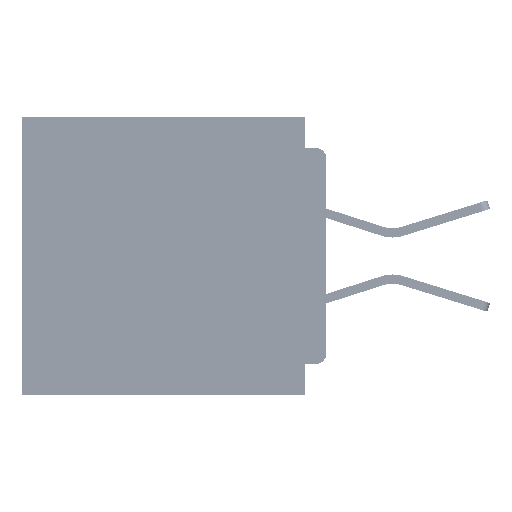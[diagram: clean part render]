
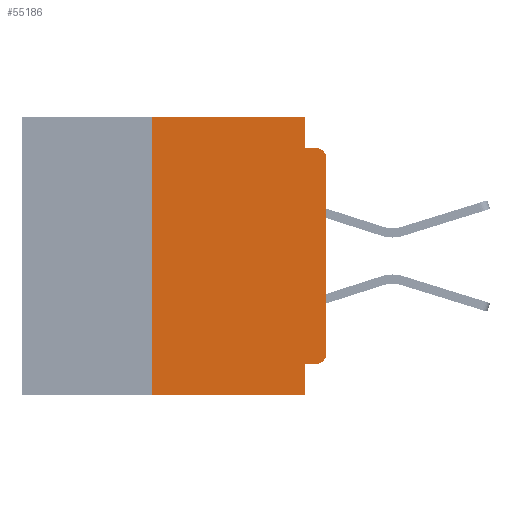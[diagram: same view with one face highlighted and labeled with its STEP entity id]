
A CAD part, left-side view. The second image highlights one B-rep face of the part: STEP entity #55186.
In plain terms, the highlighted planar face has unit normal (-1, 0, 0).
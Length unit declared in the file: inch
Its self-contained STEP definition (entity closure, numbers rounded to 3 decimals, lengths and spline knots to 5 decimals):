
#469 = EDGE_CURVE ( 'NONE', #53660, #41227, #53761, .T. ) ;
#1342 = VECTOR ( 'NONE', #25049, 39.37008 ) ;
#2038 = CARTESIAN_POINT ( 'NONE',  ( 0., 0.437, -0.4 ) ) ;
#2391 = CIRCLE ( 'NONE', #58798, 0.015 ) ;
#3403 = CIRCLE ( 'NONE', #19896, 0.015 ) ;
#4155 = DIRECTION ( 'NONE',  ( 0., -1., 0. ) ) ;
#5363 = ORIENTED_EDGE ( 'NONE', *, *, #34913, .F. ) ;
#6314 = DIRECTION ( 'NONE',  ( 1., 0., 0. ) ) ;
#6345 = ORIENTED_EDGE ( 'NONE', *, *, #62724, .F. ) ;
#6368 = VERTEX_POINT ( 'NONE', #53096 ) ;
#8986 = VERTEX_POINT ( 'NONE', #53645 ) ;
#13314 = CARTESIAN_POINT ( 'NONE',  ( 0., 0.015, -0.045 ) ) ;
#13332 = ORIENTED_EDGE ( 'NONE', *, *, #47112, .T. ) ;
#13909 = CARTESIAN_POINT ( 'NONE',  ( 0., 0.437, 0. ) ) ;
#14519 = DIRECTION ( 'NONE',  ( -1., 0., 0. ) ) ;
#14532 = LINE ( 'NONE', #15084, #1342 ) ;
#15084 = CARTESIAN_POINT ( 'NONE',  ( 0., 0., -0.355 ) ) ;
#15087 = VECTOR ( 'NONE', #4155, 39.37008 ) ;
#15425 = DIRECTION ( 'NONE',  ( -1., 0., 0. ) ) ;
#15692 = LINE ( 'NONE', #61368, #55164 ) ;
#17556 = DIRECTION ( 'NONE',  ( 0., 0., -1. ) ) ;
#18637 = ORIENTED_EDGE ( 'NONE', *, *, #59738, .F. ) ;
#18730 = EDGE_CURVE ( 'NONE', #46755, #45138, #43932, .T. ) ;
#19000 = LINE ( 'NONE', #20740, #43807 ) ;
#19896 = AXIS2_PLACEMENT_3D ( 'NONE', #44179, #14519, #49122 ) ;
#20205 = AXIS2_PLACEMENT_3D ( 'NONE', #35930, #6314, #40915 ) ;
#20740 = CARTESIAN_POINT ( 'NONE',  ( 0., 0.031, -0.4 ) ) ;
#21092 = ORIENTED_EDGE ( 'NONE', *, *, #18730, .T. ) ;
#21285 = EDGE_CURVE ( 'NONE', #45138, #56382, #3403, .T. ) ;
#21872 = DIRECTION ( 'NONE',  ( 0., -1., 0. ) ) ;
#21956 = CARTESIAN_POINT ( 'NONE',  ( 0., 0.031, -0.4 ) ) ;
#22023 = VECTOR ( 'NONE', #17556, 39.37008 ) ;
#22324 = EDGE_CURVE ( 'NONE', #53660, #56052, #59729, .T. ) ;
#23099 = DIRECTION ( 'NONE',  ( 0., 0., 1. ) ) ;
#25049 = DIRECTION ( 'NONE',  ( 0., 1., 0. ) ) ;
#25696 = CARTESIAN_POINT ( 'NONE',  ( 0., 0.25, 0. ) ) ;
#25721 = DIRECTION ( 'NONE',  ( 0., 0., -1. ) ) ;
#26771 = DIRECTION ( 'NONE',  ( 0., -1., 0. ) ) ;
#27469 = VECTOR ( 'NONE', #26771, 39.37008 ) ;
#28266 = LINE ( 'NONE', #13909, #15087 ) ;
#29336 = CARTESIAN_POINT ( 'NONE',  ( 0., 0.031, -0.045 ) ) ;
#30130 = CARTESIAN_POINT ( 'NONE',  ( 0., 0., 0. ) ) ;
#30269 = ORIENTED_EDGE ( 'NONE', *, *, #53497, .F. ) ;
#31721 = FACE_OUTER_BOUND ( 'NONE', #54273, .T. ) ;
#33463 = VECTOR ( 'NONE', #23099, 39.37008 ) ;
#34913 = EDGE_CURVE ( 'NONE', #56052, #39767, #28266, .T. ) ;
#35061 = DIRECTION ( 'NONE',  ( 0., 0., 1. ) ) ;
#35141 = LINE ( 'NONE', #42232, #22023 ) ;
#35930 = CARTESIAN_POINT ( 'NONE',  ( 0., 0.437, 0. ) ) ;
#36572 = ORIENTED_EDGE ( 'NONE', *, *, #48236, .F. ) ;
#39767 = VERTEX_POINT ( 'NONE', #54332 ) ;
#40791 = VECTOR ( 'NONE', #35061, 39.37008 ) ;
#40915 = DIRECTION ( 'NONE',  ( 0., 0., -1. ) ) ;
#41227 = VERTEX_POINT ( 'NONE', #21956 ) ;
#42232 = CARTESIAN_POINT ( 'NONE',  ( 0., 0.031, 0. ) ) ;
#43361 = CARTESIAN_POINT ( 'NONE',  ( 0., 0., -0.06 ) ) ;
#43807 = VECTOR ( 'NONE', #25721, 39.37008 ) ;
#43932 = LINE ( 'NONE', #30130, #40791 ) ;
#44179 = CARTESIAN_POINT ( 'NONE',  ( 0., 0.015, -0.06 ) ) ;
#45079 = CARTESIAN_POINT ( 'NONE',  ( 0., 0.015, -0.34 ) ) ;
#45138 = VERTEX_POINT ( 'NONE', #43361 ) ;
#45857 = ORIENTED_EDGE ( 'NONE', *, *, #22324, .F. ) ;
#46755 = VERTEX_POINT ( 'NONE', #51128 ) ;
#47112 = EDGE_CURVE ( 'NONE', #8986, #46755, #2391, .T. ) ;
#48236 = EDGE_CURVE ( 'NONE', #8986, #6368, #14532, .T. ) ;
#49122 = DIRECTION ( 'NONE',  ( 0., 0., -1. ) ) ;
#50049 = DIRECTION ( 'NONE',  ( 0., 0., -1. ) ) ;
#50784 = ORIENTED_EDGE ( 'NONE', *, *, #469, .T. ) ;
#51128 = CARTESIAN_POINT ( 'NONE',  ( 0., 0., -0.34 ) ) ;
#52140 = VERTEX_POINT ( 'NONE', #29336 ) ;
#52689 = CARTESIAN_POINT ( 'NONE',  ( 0., 0.25, -0.4 ) ) ;
#53096 = CARTESIAN_POINT ( 'NONE',  ( 0., 0.031, -0.355 ) ) ;
#53497 = EDGE_CURVE ( 'NONE', #52140, #56382, #15692, .T. ) ;
#53645 = CARTESIAN_POINT ( 'NONE',  ( 0., 0.015, -0.355 ) ) ;
#53660 = VERTEX_POINT ( 'NONE', #62606 ) ;
#53761 = LINE ( 'NONE', #2038, #27469 ) ;
#54273 = EDGE_LOOP ( 'NONE', ( #21092, #62922, #30269, #18637, #5363, #45857, #50784, #6345, #36572, #13332 ) ) ;
#54332 = CARTESIAN_POINT ( 'NONE',  ( 0., 0.031, 0. ) ) ;
#55164 = VECTOR ( 'NONE', #21872, 39.37008 ) ;
#55186 = ADVANCED_FACE ( 'NONE', ( #31721 ), #55413, .F. ) ;
#55413 = PLANE ( 'NONE',  #20205 ) ;
#56052 = VERTEX_POINT ( 'NONE', #25696 ) ;
#56382 = VERTEX_POINT ( 'NONE', #13314 ) ;
#58798 = AXIS2_PLACEMENT_3D ( 'NONE', #45079, #15425, #50049 ) ;
#59729 = LINE ( 'NONE', #52689, #33463 ) ;
#59738 = EDGE_CURVE ( 'NONE', #39767, #52140, #35141, .T. ) ;
#61368 = CARTESIAN_POINT ( 'NONE',  ( 0., 0., -0.045 ) ) ;
#62606 = CARTESIAN_POINT ( 'NONE',  ( 0., 0.25, -0.4 ) ) ;
#62724 = EDGE_CURVE ( 'NONE', #6368, #41227, #19000, .T. ) ;
#62922 = ORIENTED_EDGE ( 'NONE', *, *, #21285, .T. ) ;
